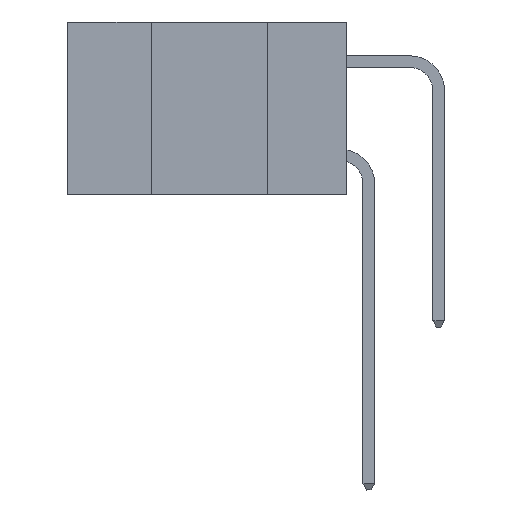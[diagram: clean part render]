
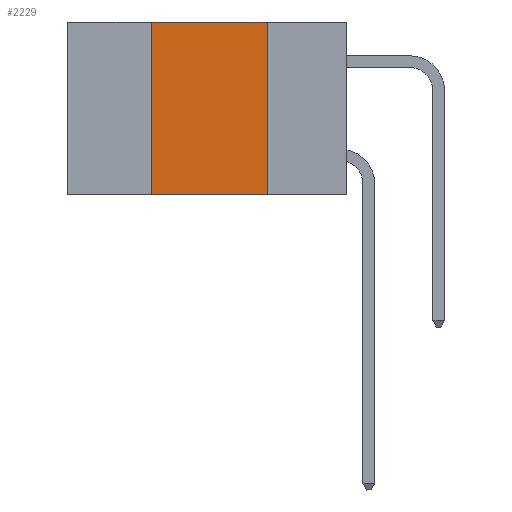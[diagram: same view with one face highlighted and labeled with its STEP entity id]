
A CAD part, left-side view. The second image highlights one B-rep face of the part: STEP entity #2229.
In plain terms, the highlighted planar face has unit normal (-1, 0, 0).
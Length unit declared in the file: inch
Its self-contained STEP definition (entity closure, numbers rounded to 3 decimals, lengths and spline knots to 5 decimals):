
#96 = LINE ( 'NONE', #29209, #29404 ) ;
#973 = VECTOR ( 'NONE', #32520, 39.37008 ) ;
#1244 = VECTOR ( 'NONE', #34193, 39.37008 ) ;
#1517 = ORIENTED_EDGE ( 'NONE', *, *, #17538, .F. ) ;
#2229 = ADVANCED_FACE ( 'NONE', ( #14953 ), #5526, .F. ) ;
#3155 = LINE ( 'NONE', #25594, #33281 ) ;
#3789 = VERTEX_POINT ( 'NONE', #20682 ) ;
#3958 = AXIS2_PLACEMENT_3D ( 'NONE', #36599, #28350, #11445 ) ;
#4596 = LINE ( 'NONE', #18472, #973 ) ;
#5487 = VERTEX_POINT ( 'NONE', #18990 ) ;
#5526 = PLANE ( 'NONE',  #3958 ) ;
#7918 = VERTEX_POINT ( 'NONE', #15602 ) ;
#7951 = EDGE_CURVE ( 'NONE', #5487, #7918, #4596, .T. ) ;
#8577 = DIRECTION ( 'NONE',  ( 0., -1., 0. ) ) ;
#8904 = LINE ( 'NONE', #31420, #1244 ) ;
#9650 = ORIENTED_EDGE ( 'NONE', *, *, #22920, .T. ) ;
#11445 = DIRECTION ( 'NONE',  ( 0., 0., -1. ) ) ;
#13135 = EDGE_CURVE ( 'NONE', #7918, #22564, #8904, .T. ) ;
#14572 = ORIENTED_EDGE ( 'NONE', *, *, #7951, .F. ) ;
#14953 = FACE_OUTER_BOUND ( 'NONE', #15320, .T. ) ;
#15320 = EDGE_LOOP ( 'NONE', ( #1517, #36047, #14572, #9650 ) ) ;
#15602 = CARTESIAN_POINT ( 'NONE',  ( 0., 0.42, 0. ) ) ;
#17538 = EDGE_CURVE ( 'NONE', #22564, #3789, #96, .T. ) ;
#18472 = CARTESIAN_POINT ( 'NONE',  ( 0., 0.42, 0. ) ) ;
#18990 = CARTESIAN_POINT ( 'NONE',  ( 0., 0.42, -0.37 ) ) ;
#20682 = CARTESIAN_POINT ( 'NONE',  ( 0., 0.17, -0.37 ) ) ;
#22564 = VERTEX_POINT ( 'NONE', #32292 ) ;
#22920 = EDGE_CURVE ( 'NONE', #5487, #3789, #3155, .T. ) ;
#23635 = DIRECTION ( 'NONE',  ( 0., 0., -1. ) ) ;
#25594 = CARTESIAN_POINT ( 'NONE',  ( 0., 0.6, -0.37 ) ) ;
#28350 = DIRECTION ( 'NONE',  ( 1., 0., 0. ) ) ;
#29209 = CARTESIAN_POINT ( 'NONE',  ( 0., 0.17, 0. ) ) ;
#29404 = VECTOR ( 'NONE', #23635, 39.37008 ) ;
#31420 = CARTESIAN_POINT ( 'NONE',  ( 0., 0.6, 0. ) ) ;
#32292 = CARTESIAN_POINT ( 'NONE',  ( 0., 0.17, 0. ) ) ;
#32520 = DIRECTION ( 'NONE',  ( 0., 0., 1. ) ) ;
#33281 = VECTOR ( 'NONE', #8577, 39.37008 ) ;
#34193 = DIRECTION ( 'NONE',  ( 0., -1., 0. ) ) ;
#36047 = ORIENTED_EDGE ( 'NONE', *, *, #13135, .F. ) ;
#36599 = CARTESIAN_POINT ( 'NONE',  ( 0., 0.6, 0. ) ) ;
